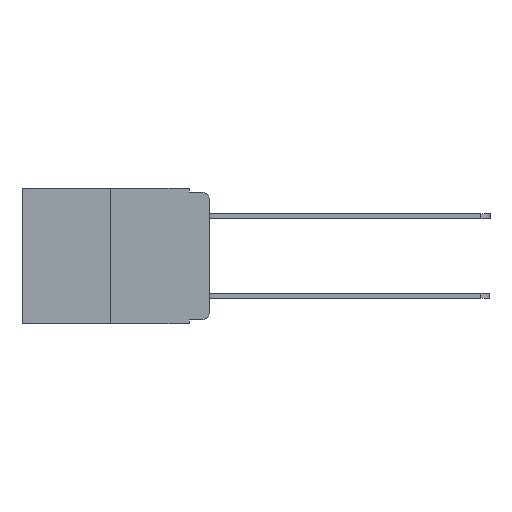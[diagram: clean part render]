
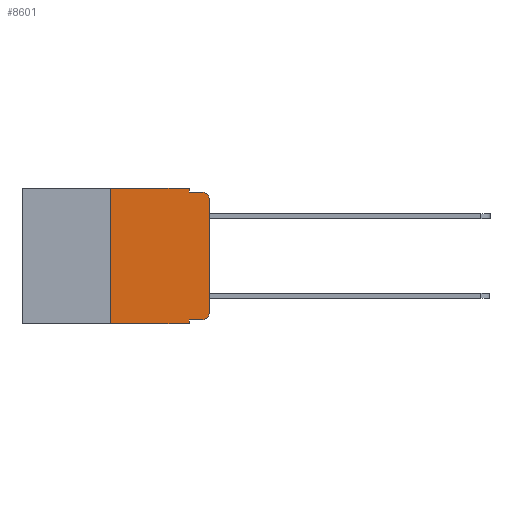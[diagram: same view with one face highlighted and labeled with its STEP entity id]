
A CAD part, left-side view. The second image highlights one B-rep face of the part: STEP entity #8601.
In plain terms, the highlighted planar face has unit normal (-1, 0, 0).
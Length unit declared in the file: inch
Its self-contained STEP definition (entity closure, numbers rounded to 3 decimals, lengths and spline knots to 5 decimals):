
#58 = VERTEX_POINT ( 'NONE', #8187 ) ;
#202 = DIRECTION ( 'NONE',  ( 0., 0., -1. ) ) ;
#265 = LINE ( 'NONE', #12832, #8785 ) ;
#316 = EDGE_CURVE ( 'NONE', #7390, #11871, #6735, .T. ) ;
#508 = DIRECTION ( 'NONE',  ( 0., 0., 1. ) ) ;
#567 = CIRCLE ( 'NONE', #11682, 0.02 ) ;
#622 = VECTOR ( 'NONE', #3073, 39.37008 ) ;
#667 = CARTESIAN_POINT ( 'NONE',  ( 0., 0.051, 0. ) ) ;
#716 = VERTEX_POINT ( 'NONE', #10183 ) ;
#718 = PLANE ( 'NONE',  #3988 ) ;
#1686 = AXIS2_PLACEMENT_3D ( 'NONE', #11276, #5441, #12217 ) ;
#1713 = CARTESIAN_POINT ( 'NONE',  ( 0., 0.25, 0. ) ) ;
#1802 = VECTOR ( 'NONE', #508, 39.37008 ) ;
#1976 = VERTEX_POINT ( 'NONE', #9062 ) ;
#1984 = DIRECTION ( 'NONE',  ( 1., 0., 0. ) ) ;
#2229 = ORIENTED_EDGE ( 'NONE', *, *, #9318, .F. ) ;
#3073 = DIRECTION ( 'NONE',  ( 0., 0., 1. ) ) ;
#3216 = CARTESIAN_POINT ( 'NONE',  ( 0., 0.473, 0. ) ) ;
#3389 = CARTESIAN_POINT ( 'NONE',  ( 0., 0.473, -0.343 ) ) ;
#3448 = CARTESIAN_POINT ( 'NONE',  ( 0., 0.051, -0.01 ) ) ;
#3492 = VERTEX_POINT ( 'NONE', #4378 ) ;
#3636 = DIRECTION ( 'NONE',  ( 0., -1., 0. ) ) ;
#3757 = EDGE_CURVE ( 'NONE', #58, #716, #567, .T. ) ;
#3958 = CARTESIAN_POINT ( 'NONE',  ( 0., 0.051, 0. ) ) ;
#3988 = AXIS2_PLACEMENT_3D ( 'NONE', #13213, #1984, #9458 ) ;
#4054 = DIRECTION ( 'NONE',  ( -1., 0., 0. ) ) ;
#4378 = CARTESIAN_POINT ( 'NONE',  ( 0., 0.051, -0.343 ) ) ;
#4387 = CARTESIAN_POINT ( 'NONE',  ( 0., 0.02, -0.01 ) ) ;
#5040 = DIRECTION ( 'NONE',  ( 0., -1., 0. ) ) ;
#5174 = VERTEX_POINT ( 'NONE', #10554 ) ;
#5355 = EDGE_CURVE ( 'NONE', #1976, #58, #265, .T. ) ;
#5441 = DIRECTION ( 'NONE',  ( -1., 0., 0. ) ) ;
#5445 = ORIENTED_EDGE ( 'NONE', *, *, #3757, .T. ) ;
#5589 = ORIENTED_EDGE ( 'NONE', *, *, #316, .F. ) ;
#6037 = EDGE_CURVE ( 'NONE', #1976, #3492, #10121, .T. ) ;
#6213 = DIRECTION ( 'NONE',  ( 0., 0., -1. ) ) ;
#6244 = EDGE_LOOP ( 'NONE', ( #8507, #11358, #12512, #2229, #5589, #6838, #7757, #8675, #6552, #5445 ) ) ;
#6552 = ORIENTED_EDGE ( 'NONE', *, *, #5355, .T. ) ;
#6735 = LINE ( 'NONE', #3216, #11840 ) ;
#6747 = DIRECTION ( 'NONE',  ( 0., -1., 0. ) ) ;
#6838 = ORIENTED_EDGE ( 'NONE', *, *, #7381, .F. ) ;
#6914 = LINE ( 'NONE', #13395, #9191 ) ;
#7381 = EDGE_CURVE ( 'NONE', #9905, #7390, #7398, .T. ) ;
#7390 = VERTEX_POINT ( 'NONE', #8342 ) ;
#7398 = LINE ( 'NONE', #1713, #1802 ) ;
#7757 = ORIENTED_EDGE ( 'NONE', *, *, #8828, .T. ) ;
#7842 = VECTOR ( 'NONE', #6747, 39.37008 ) ;
#8092 = CARTESIAN_POINT ( 'NONE',  ( 0., 0.051, 0. ) ) ;
#8187 = CARTESIAN_POINT ( 'NONE',  ( 0., 0.02, -0.333 ) ) ;
#8342 = CARTESIAN_POINT ( 'NONE',  ( 0., 0.25, 0. ) ) ;
#8507 = ORIENTED_EDGE ( 'NONE', *, *, #11872, .T. ) ;
#8601 = ADVANCED_FACE ( 'NONE', ( #9061 ), #718, .F. ) ;
#8611 = VERTEX_POINT ( 'NONE', #4387 ) ;
#8675 = ORIENTED_EDGE ( 'NONE', *, *, #6037, .F. ) ;
#8785 = VECTOR ( 'NONE', #5040, 39.37008 ) ;
#8828 = EDGE_CURVE ( 'NONE', #9905, #3492, #10410, .T. ) ;
#8913 = VERTEX_POINT ( 'NONE', #3448 ) ;
#9061 = FACE_OUTER_BOUND ( 'NONE', #6244, .T. ) ;
#9062 = CARTESIAN_POINT ( 'NONE',  ( 0., 0.051, -0.333 ) ) ;
#9191 = VECTOR ( 'NONE', #12462, 39.37008 ) ;
#9318 = EDGE_CURVE ( 'NONE', #11871, #8913, #10552, .T. ) ;
#9360 = LINE ( 'NONE', #13166, #622 ) ;
#9458 = DIRECTION ( 'NONE',  ( 0., 0., -1. ) ) ;
#9566 = CARTESIAN_POINT ( 'NONE',  ( 0., 0.25, -0.343 ) ) ;
#9905 = VERTEX_POINT ( 'NONE', #9566 ) ;
#9958 = EDGE_CURVE ( 'NONE', #8913, #8611, #6914, .T. ) ;
#10121 = LINE ( 'NONE', #8092, #12631 ) ;
#10142 = CARTESIAN_POINT ( 'NONE',  ( 0., 0.02, -0.313 ) ) ;
#10183 = CARTESIAN_POINT ( 'NONE',  ( 0., 0., -0.313 ) ) ;
#10239 = VECTOR ( 'NONE', #6213, 39.37008 ) ;
#10410 = LINE ( 'NONE', #3389, #7842 ) ;
#10552 = LINE ( 'NONE', #3958, #10239 ) ;
#10554 = CARTESIAN_POINT ( 'NONE',  ( 0., 0., -0.03 ) ) ;
#10601 = EDGE_CURVE ( 'NONE', #5174, #8611, #12768, .T. ) ;
#11109 = DIRECTION ( 'NONE',  ( 0., 0., -1. ) ) ;
#11276 = CARTESIAN_POINT ( 'NONE',  ( 0., 0.02, -0.03 ) ) ;
#11358 = ORIENTED_EDGE ( 'NONE', *, *, #10601, .T. ) ;
#11682 = AXIS2_PLACEMENT_3D ( 'NONE', #10142, #4054, #11109 ) ;
#11840 = VECTOR ( 'NONE', #3636, 39.37008 ) ;
#11871 = VERTEX_POINT ( 'NONE', #667 ) ;
#11872 = EDGE_CURVE ( 'NONE', #716, #5174, #9360, .T. ) ;
#12217 = DIRECTION ( 'NONE',  ( 0., 0., -1. ) ) ;
#12462 = DIRECTION ( 'NONE',  ( 0., -1., 0. ) ) ;
#12512 = ORIENTED_EDGE ( 'NONE', *, *, #9958, .F. ) ;
#12631 = VECTOR ( 'NONE', #202, 39.37008 ) ;
#12768 = CIRCLE ( 'NONE', #1686, 0.02 ) ;
#12832 = CARTESIAN_POINT ( 'NONE',  ( 0., 0.051, -0.333 ) ) ;
#13166 = CARTESIAN_POINT ( 'NONE',  ( 0., 0., 0. ) ) ;
#13213 = CARTESIAN_POINT ( 'NONE',  ( 0., 0.473, 0. ) ) ;
#13395 = CARTESIAN_POINT ( 'NONE',  ( 0., 0.051, -0.01 ) ) ;
